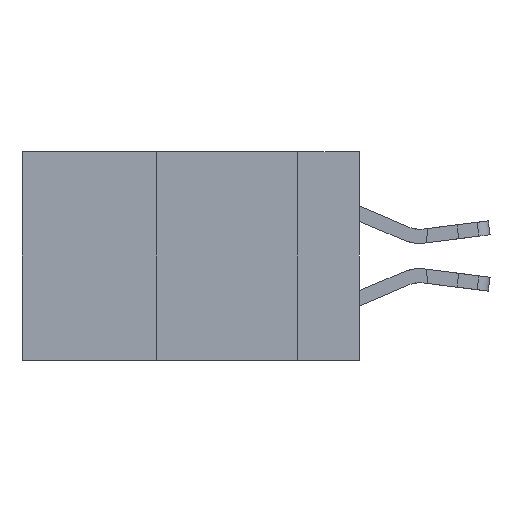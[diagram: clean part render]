
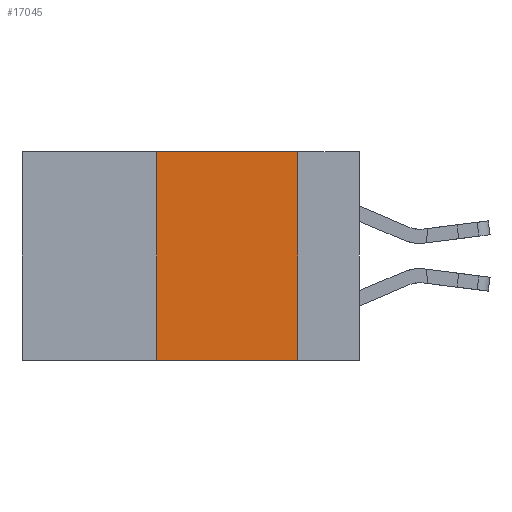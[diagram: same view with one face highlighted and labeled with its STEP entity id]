
A CAD part, left-side view. The second image highlights one B-rep face of the part: STEP entity #17045.
In plain terms, the highlighted planar face has unit normal (-1, 0, 0).
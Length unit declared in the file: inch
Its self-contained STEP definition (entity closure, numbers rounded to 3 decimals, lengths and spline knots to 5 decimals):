
#142 = VERTEX_POINT ( 'NONE', #14658 ) ;
#182 = LINE ( 'NONE', #14718, #9414 ) ;
#790 = PLANE ( 'NONE',  #14780 ) ;
#966 = ORIENTED_EDGE ( 'NONE', *, *, #14441, .T. ) ;
#1812 = DIRECTION ( 'NONE',  ( 0., 0., 1. ) ) ;
#2066 = CARTESIAN_POINT ( 'NONE',  ( 0., 0.6, -0.37 ) ) ;
#2854 = LINE ( 'NONE', #17630, #16314 ) ;
#3588 = DIRECTION ( 'NONE',  ( 0., 0., -1. ) ) ;
#3663 = VECTOR ( 'NONE', #1812, 39.37008 ) ;
#3817 = VERTEX_POINT ( 'NONE', #7886 ) ;
#5549 = FACE_OUTER_BOUND ( 'NONE', #15405, .T. ) ;
#5568 = VERTEX_POINT ( 'NONE', #13750 ) ;
#5871 = VECTOR ( 'NONE', #8979, 39.37008 ) ;
#7313 = CARTESIAN_POINT ( 'NONE',  ( 0., 0.36, 0. ) ) ;
#7742 = LINE ( 'NONE', #7313, #3663 ) ;
#7886 = CARTESIAN_POINT ( 'NONE',  ( 0., 0.11, 0. ) ) ;
#8463 = VERTEX_POINT ( 'NONE', #12844 ) ;
#8979 = DIRECTION ( 'NONE',  ( 0., -1., 0. ) ) ;
#9414 = VECTOR ( 'NONE', #16268, 39.37008 ) ;
#9495 = LINE ( 'NONE', #2066, #5871 ) ;
#9716 = EDGE_CURVE ( 'NONE', #5568, #3817, #2854, .T. ) ;
#10602 = ORIENTED_EDGE ( 'NONE', *, *, #9716, .F. ) ;
#10873 = DIRECTION ( 'NONE',  ( 0., -1., 0. ) ) ;
#11148 = EDGE_CURVE ( 'NONE', #142, #5568, #7742, .T. ) ;
#12844 = CARTESIAN_POINT ( 'NONE',  ( 0., 0.11, -0.37 ) ) ;
#13178 = CARTESIAN_POINT ( 'NONE',  ( 0., 0.6, 0. ) ) ;
#13750 = CARTESIAN_POINT ( 'NONE',  ( 0., 0.36, 0. ) ) ;
#14441 = EDGE_CURVE ( 'NONE', #142, #8463, #9495, .T. ) ;
#14658 = CARTESIAN_POINT ( 'NONE',  ( 0., 0.36, -0.37 ) ) ;
#14718 = CARTESIAN_POINT ( 'NONE',  ( 0., 0.11, 0. ) ) ;
#14780 = AXIS2_PLACEMENT_3D ( 'NONE', #13178, #15924, #3588 ) ;
#15087 = ORIENTED_EDGE ( 'NONE', *, *, #15929, .F. ) ;
#15405 = EDGE_LOOP ( 'NONE', ( #15087, #10602, #15493, #966 ) ) ;
#15493 = ORIENTED_EDGE ( 'NONE', *, *, #11148, .F. ) ;
#15924 = DIRECTION ( 'NONE',  ( 1., 0., 0. ) ) ;
#15929 = EDGE_CURVE ( 'NONE', #3817, #8463, #182, .T. ) ;
#16268 = DIRECTION ( 'NONE',  ( 0., 0., -1. ) ) ;
#16314 = VECTOR ( 'NONE', #10873, 39.37008 ) ;
#17045 = ADVANCED_FACE ( 'NONE', ( #5549 ), #790, .F. ) ;
#17630 = CARTESIAN_POINT ( 'NONE',  ( 0., 0.6, 0. ) ) ;
